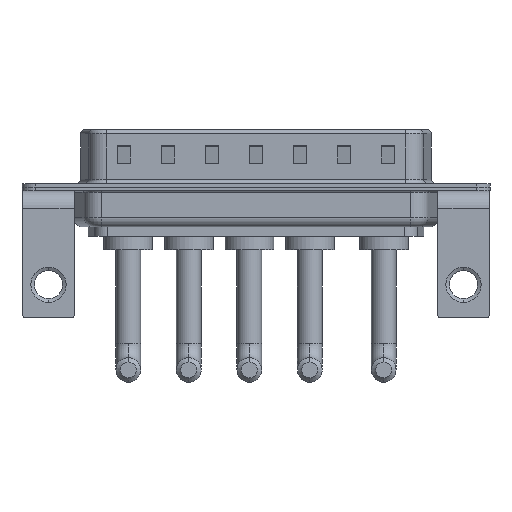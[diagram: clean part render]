
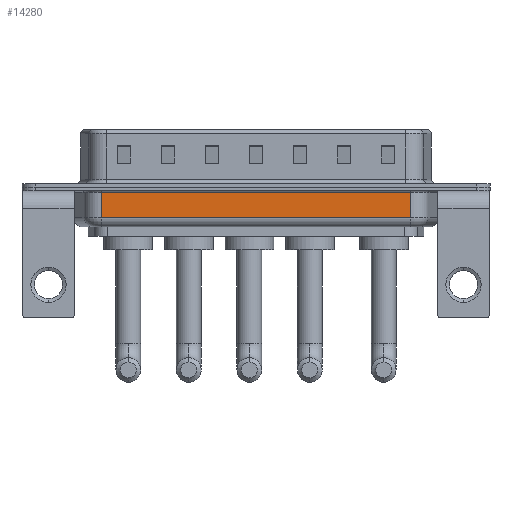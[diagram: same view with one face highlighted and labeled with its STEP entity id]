
A CAD part, front view. The second image highlights one B-rep face of the part: STEP entity #14280.
In plain terms, the highlighted planar face has unit normal (0, -1, 0).
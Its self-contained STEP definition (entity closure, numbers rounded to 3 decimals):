
#44 = EDGE_CURVE ( 'NONE', #57, #12201, #6120, .T. ) ;
#57 = VERTEX_POINT ( 'NONE', #12948 ) ;
#215 = DIRECTION ( 'NONE',  ( -1., 0., 0. ) ) ;
#1717 = CARTESIAN_POINT ( 'NONE',  ( 6.006, -5.35, -0.65 ) ) ;
#1922 = CARTESIAN_POINT ( 'NONE',  ( 6.006, -5.35, -3.5 ) ) ;
#2349 = DIRECTION ( 'NONE',  ( 0., 0., 1. ) ) ;
#2467 = ORIENTED_EDGE ( 'NONE', *, *, #12439, .T. ) ;
#2718 = VERTEX_POINT ( 'NONE', #12702 ) ;
#2760 = DIRECTION ( 'NONE',  ( 0., 0., 1. ) ) ;
#2890 = ORIENTED_EDGE ( 'NONE', *, *, #44, .T. ) ;
#3378 = LINE ( 'NONE', #14011, #11778 ) ;
#3543 = ORIENTED_EDGE ( 'NONE', *, *, #13334, .T. ) ;
#3827 = DIRECTION ( 'NONE',  ( 0., 0., 1. ) ) ;
#3865 = CARTESIAN_POINT ( 'NONE',  ( 6.006, -5.35, -0.65 ) ) ;
#4285 = EDGE_CURVE ( 'NONE', #10250, #12201, #13537, .T. ) ;
#5486 = CARTESIAN_POINT ( 'NONE',  ( 6.006, -5.35, -3.5 ) ) ;
#6120 = LINE ( 'NONE', #3865, #13793 ) ;
#10063 = LINE ( 'NONE', #5486, #10564 ) ;
#10092 = AXIS2_PLACEMENT_3D ( 'NONE', #11399, #13362, #3827 ) ;
#10167 = PLANE ( 'NONE',  #10092 ) ;
#10250 = VERTEX_POINT ( 'NONE', #1922 ) ;
#10564 = VECTOR ( 'NONE', #12534, 1000. ) ;
#10670 = VECTOR ( 'NONE', #2760, 1000. ) ;
#11283 = CARTESIAN_POINT ( 'NONE',  ( 6.006, -5.35, -4.5 ) ) ;
#11399 = CARTESIAN_POINT ( 'NONE',  ( 6.006, -5.35, -4.5 ) ) ;
#11778 = VECTOR ( 'NONE', #2349, 1000. ) ;
#12201 = VERTEX_POINT ( 'NONE', #1717 ) ;
#12439 = EDGE_CURVE ( 'NONE', #2718, #57, #3378, .T. ) ;
#12534 = DIRECTION ( 'NONE',  ( 1., 0., 0. ) ) ;
#12702 = CARTESIAN_POINT ( 'NONE',  ( 41.044, -5.35, -3.5 ) ) ;
#12948 = CARTESIAN_POINT ( 'NONE',  ( 41.044, -5.35, -0.65 ) ) ;
#13334 = EDGE_CURVE ( 'NONE', #10250, #2718, #10063, .T. ) ;
#13362 = DIRECTION ( 'NONE',  ( 0., 1., 0. ) ) ;
#13537 = LINE ( 'NONE', #11283, #10670 ) ;
#13793 = VECTOR ( 'NONE', #215, 1000. ) ;
#13831 = EDGE_LOOP ( 'NONE', ( #13892, #3543, #2467, #2890 ) ) ;
#13892 = ORIENTED_EDGE ( 'NONE', *, *, #4285, .F. ) ;
#14011 = CARTESIAN_POINT ( 'NONE',  ( 41.044, -5.35, -4.5 ) ) ;
#14280 = ADVANCED_FACE ( 'NONE', ( #14899 ), #10167, .F. ) ;
#14899 = FACE_OUTER_BOUND ( 'NONE', #13831, .T. ) ;
